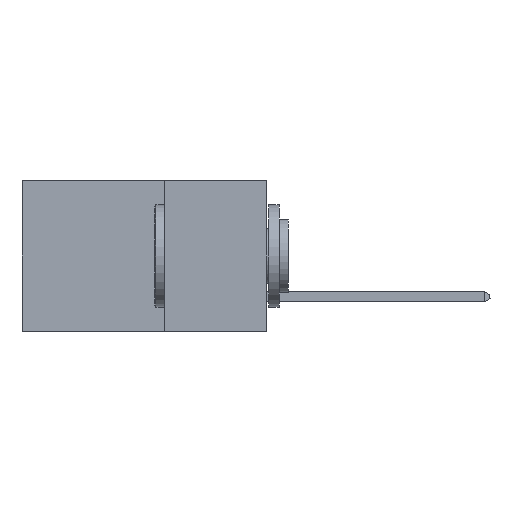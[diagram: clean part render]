
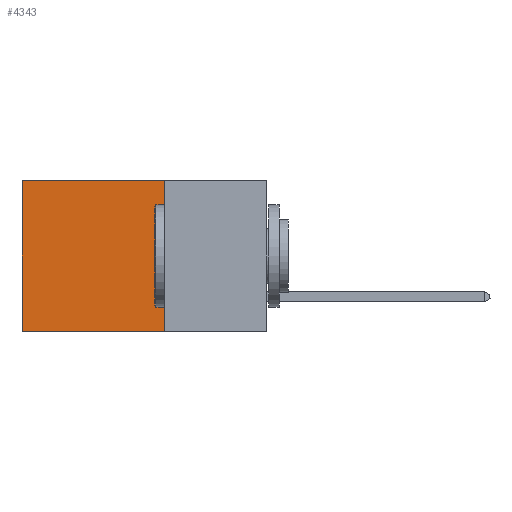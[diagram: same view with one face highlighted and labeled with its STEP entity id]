
A CAD part, left-side view. The second image highlights one B-rep face of the part: STEP entity #4343.
In plain terms, the highlighted planar face has unit normal (-1, 0, 0).
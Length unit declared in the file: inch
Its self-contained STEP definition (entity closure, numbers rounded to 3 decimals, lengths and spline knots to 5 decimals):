
#3693 = VECTOR ( 'NONE', #17723, 39.37008 ) ;
#3973 = CARTESIAN_POINT ( 'NONE',  ( 0.2875, 0.25, -0.37 ) ) ;
#4343 = ADVANCED_FACE ( 'NONE', ( #35784 ), #24935, .F. ) ;
#4597 = VERTEX_POINT ( 'NONE', #15368 ) ;
#5209 = AXIS2_PLACEMENT_3D ( 'NONE', #24668, #30842, #7217 ) ;
#6051 = EDGE_CURVE ( 'NONE', #29980, #26053, #36265, .T. ) ;
#7217 = DIRECTION ( 'NONE',  ( 0., 0., -1. ) ) ;
#8513 = DIRECTION ( 'NONE',  ( 0., 1., 0. ) ) ;
#8595 = EDGE_LOOP ( 'NONE', ( #9817, #34896, #27363, #31709 ) ) ;
#9028 = CARTESIAN_POINT ( 'NONE',  ( 0.2875, 0.25, 0. ) ) ;
#9817 = ORIENTED_EDGE ( 'NONE', *, *, #16331, .T. ) ;
#11463 = LINE ( 'NONE', #12329, #3693 ) ;
#12247 = EDGE_CURVE ( 'NONE', #4597, #25976, #11463, .T. ) ;
#12329 = CARTESIAN_POINT ( 'NONE',  ( 0.2875, 0.25, 0. ) ) ;
#15317 = LINE ( 'NONE', #9028, #33102 ) ;
#15368 = CARTESIAN_POINT ( 'NONE',  ( 0.2875, 0.25, 0. ) ) ;
#16065 = EDGE_CURVE ( 'NONE', #4597, #29980, #15317, .T. ) ;
#16331 = EDGE_CURVE ( 'NONE', #25976, #26053, #19446, .T. ) ;
#17565 = VECTOR ( 'NONE', #8513, 39.37008 ) ;
#17723 = DIRECTION ( 'NONE',  ( 0., 1., 0. ) ) ;
#19446 = LINE ( 'NONE', #21304, #27190 ) ;
#20031 = CARTESIAN_POINT ( 'NONE',  ( 0.2875, 0.6, 0. ) ) ;
#21304 = CARTESIAN_POINT ( 'NONE',  ( 0.2875, 0.6, 0. ) ) ;
#23554 = CARTESIAN_POINT ( 'NONE',  ( 0.2875, 0.6, -0.37 ) ) ;
#24668 = CARTESIAN_POINT ( 'NONE',  ( 0.2875, 0.25, 0. ) ) ;
#24935 = PLANE ( 'NONE',  #5209 ) ;
#25976 = VERTEX_POINT ( 'NONE', #20031 ) ;
#25983 = CARTESIAN_POINT ( 'NONE',  ( 0.2875, 0.25, -0.37 ) ) ;
#26053 = VERTEX_POINT ( 'NONE', #23554 ) ;
#27190 = VECTOR ( 'NONE', #33189, 39.37008 ) ;
#27363 = ORIENTED_EDGE ( 'NONE', *, *, #16065, .F. ) ;
#29980 = VERTEX_POINT ( 'NONE', #3973 ) ;
#30842 = DIRECTION ( 'NONE',  ( 1., 0., 0. ) ) ;
#31709 = ORIENTED_EDGE ( 'NONE', *, *, #12247, .T. ) ;
#32535 = DIRECTION ( 'NONE',  ( 0., 0., -1. ) ) ;
#33102 = VECTOR ( 'NONE', #32535, 39.37008 ) ;
#33189 = DIRECTION ( 'NONE',  ( 0., 0., -1. ) ) ;
#34896 = ORIENTED_EDGE ( 'NONE', *, *, #6051, .F. ) ;
#35784 = FACE_OUTER_BOUND ( 'NONE', #8595, .T. ) ;
#36265 = LINE ( 'NONE', #25983, #17565 ) ;
